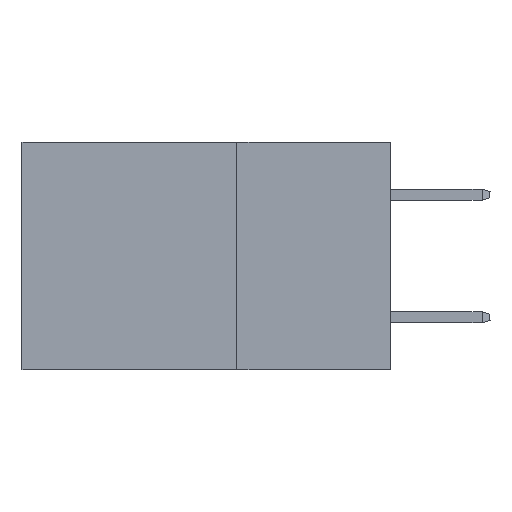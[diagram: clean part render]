
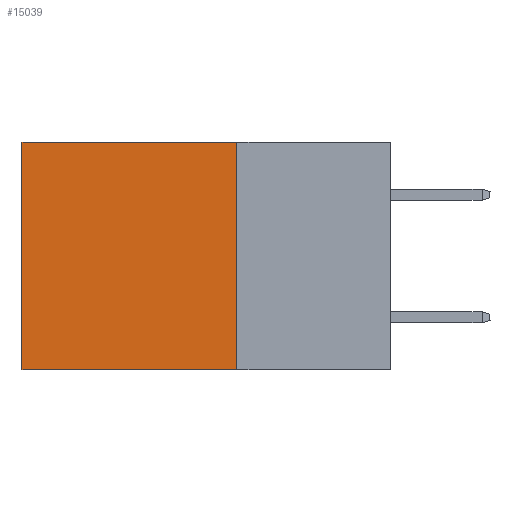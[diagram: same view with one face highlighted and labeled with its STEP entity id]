
A CAD part, left-side view. The second image highlights one B-rep face of the part: STEP entity #15039.
In plain terms, the highlighted planar face has unit normal (-1, 0, 0).
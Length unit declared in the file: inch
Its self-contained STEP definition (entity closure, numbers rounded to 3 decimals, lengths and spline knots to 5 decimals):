
#933 = ORIENTED_EDGE ( 'NONE', *, *, #17275, .T. ) ;
#943 = EDGE_CURVE ( 'NONE', #16069, #2116, #18347, .T. ) ;
#1036 = VECTOR ( 'NONE', #15678, 39.37008 ) ;
#1377 = FACE_OUTER_BOUND ( 'NONE', #23596, .T. ) ;
#1980 = VECTOR ( 'NONE', #19702, 39.37008 ) ;
#2116 = VERTEX_POINT ( 'NONE', #3373 ) ;
#2246 = ORIENTED_EDGE ( 'NONE', *, *, #16473, .F. ) ;
#3373 = CARTESIAN_POINT ( 'NONE',  ( 0.2875, 0.25, -0.37 ) ) ;
#3720 = ORIENTED_EDGE ( 'NONE', *, *, #943, .F. ) ;
#4337 = CARTESIAN_POINT ( 'NONE',  ( 0.2875, 0.25, 0. ) ) ;
#5459 = CARTESIAN_POINT ( 'NONE',  ( 0.2875, 0.25, 0. ) ) ;
#6533 = CARTESIAN_POINT ( 'NONE',  ( 0.2875, 0.25, 0. ) ) ;
#7257 = LINE ( 'NONE', #4337, #12119 ) ;
#7343 = AXIS2_PLACEMENT_3D ( 'NONE', #6533, #8459, #19424 ) ;
#8459 = DIRECTION ( 'NONE',  ( 1., 0., 0. ) ) ;
#8467 = VERTEX_POINT ( 'NONE', #16720 ) ;
#9364 = ORIENTED_EDGE ( 'NONE', *, *, #11865, .T. ) ;
#11660 = VECTOR ( 'NONE', #16382, 39.37008 ) ;
#11865 = EDGE_CURVE ( 'NONE', #16069, #8467, #7257, .T. ) ;
#12024 = LINE ( 'NONE', #14145, #1980 ) ;
#12119 = VECTOR ( 'NONE', #17134, 39.37008 ) ;
#14145 = CARTESIAN_POINT ( 'NONE',  ( 0.2875, 0.6, 0. ) ) ;
#15039 = ADVANCED_FACE ( 'NONE', ( #1377 ), #17399, .F. ) ;
#15678 = DIRECTION ( 'NONE',  ( 0., 1., 0. ) ) ;
#15988 = CARTESIAN_POINT ( 'NONE',  ( 0.2875, 0.25, -0.37 ) ) ;
#16069 = VERTEX_POINT ( 'NONE', #5459 ) ;
#16382 = DIRECTION ( 'NONE',  ( 0., 0., -1. ) ) ;
#16473 = EDGE_CURVE ( 'NONE', #2116, #21923, #17150, .T. ) ;
#16611 = CARTESIAN_POINT ( 'NONE',  ( 0.2875, 0.6, -0.37 ) ) ;
#16720 = CARTESIAN_POINT ( 'NONE',  ( 0.2875, 0.6, 0. ) ) ;
#17134 = DIRECTION ( 'NONE',  ( 0., 1., 0. ) ) ;
#17150 = LINE ( 'NONE', #15988, #1036 ) ;
#17275 = EDGE_CURVE ( 'NONE', #8467, #21923, #12024, .T. ) ;
#17399 = PLANE ( 'NONE',  #7343 ) ;
#18347 = LINE ( 'NONE', #21283, #11660 ) ;
#19424 = DIRECTION ( 'NONE',  ( 0., 0., -1. ) ) ;
#19702 = DIRECTION ( 'NONE',  ( 0., 0., -1. ) ) ;
#21283 = CARTESIAN_POINT ( 'NONE',  ( 0.2875, 0.25, 0. ) ) ;
#21923 = VERTEX_POINT ( 'NONE', #16611 ) ;
#23596 = EDGE_LOOP ( 'NONE', ( #933, #2246, #3720, #9364 ) ) ;
